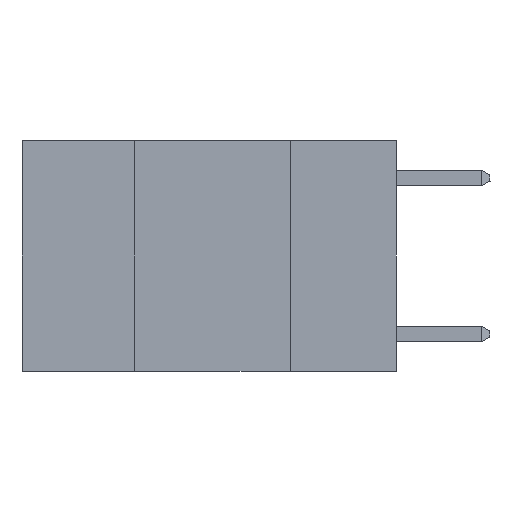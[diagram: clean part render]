
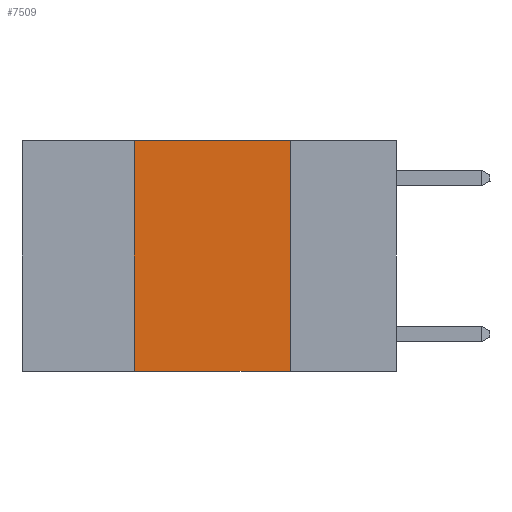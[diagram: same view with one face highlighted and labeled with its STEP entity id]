
A CAD part, left-side view. The second image highlights one B-rep face of the part: STEP entity #7509.
In plain terms, the highlighted planar face has unit normal (-1, 0, 0).
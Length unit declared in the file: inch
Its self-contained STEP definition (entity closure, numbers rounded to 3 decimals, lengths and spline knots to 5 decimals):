
#408 = ORIENTED_EDGE ( 'NONE', *, *, #969, .F. ) ;
#866 = LINE ( 'NONE', #1136, #2808 ) ;
#969 = EDGE_CURVE ( 'NONE', #2059, #5249, #866, .T. ) ;
#1136 = CARTESIAN_POINT ( 'NONE',  ( 0., 0.6, 0. ) ) ;
#1312 = AXIS2_PLACEMENT_3D ( 'NONE', #4613, #2188, #7841 ) ;
#1354 = PLANE ( 'NONE',  #1312 ) ;
#1768 = LINE ( 'NONE', #5942, #2265 ) ;
#2059 = VERTEX_POINT ( 'NONE', #3646 ) ;
#2148 = CARTESIAN_POINT ( 'NONE',  ( 0., 0.6, -0.37 ) ) ;
#2188 = DIRECTION ( 'NONE',  ( 1., 0., 0. ) ) ;
#2265 = VECTOR ( 'NONE', #7487, 39.37008 ) ;
#2636 = DIRECTION ( 'NONE',  ( 0., -1., 0. ) ) ;
#2808 = VECTOR ( 'NONE', #2636, 39.37008 ) ;
#3615 = CARTESIAN_POINT ( 'NONE',  ( 0., 0.42, -0.37 ) ) ;
#3646 = CARTESIAN_POINT ( 'NONE',  ( 0., 0.42, 0. ) ) ;
#4138 = CARTESIAN_POINT ( 'NONE',  ( 0., 0.17, 0. ) ) ;
#4613 = CARTESIAN_POINT ( 'NONE',  ( 0., 0.6, 0. ) ) ;
#5249 = VERTEX_POINT ( 'NONE', #4138 ) ;
#5309 = CARTESIAN_POINT ( 'NONE',  ( 0., 0.17, -0.37 ) ) ;
#5350 = EDGE_LOOP ( 'NONE', ( #9798, #408, #6287, #7419 ) ) ;
#5364 = EDGE_CURVE ( 'NONE', #5249, #6177, #1768, .T. ) ;
#5484 = VECTOR ( 'NONE', #7800, 39.37008 ) ;
#5546 = LINE ( 'NONE', #2148, #9553 ) ;
#5942 = CARTESIAN_POINT ( 'NONE',  ( 0., 0.17, 0. ) ) ;
#6177 = VERTEX_POINT ( 'NONE', #5309 ) ;
#6278 = EDGE_CURVE ( 'NONE', #9271, #2059, #7575, .T. ) ;
#6287 = ORIENTED_EDGE ( 'NONE', *, *, #6278, .F. ) ;
#6983 = CARTESIAN_POINT ( 'NONE',  ( 0., 0.42, 0. ) ) ;
#7419 = ORIENTED_EDGE ( 'NONE', *, *, #8772, .T. ) ;
#7487 = DIRECTION ( 'NONE',  ( 0., 0., -1. ) ) ;
#7509 = ADVANCED_FACE ( 'NONE', ( #8329 ), #1354, .F. ) ;
#7575 = LINE ( 'NONE', #6983, #5484 ) ;
#7800 = DIRECTION ( 'NONE',  ( 0., 0., 1. ) ) ;
#7841 = DIRECTION ( 'NONE',  ( 0., 0., -1. ) ) ;
#8329 = FACE_OUTER_BOUND ( 'NONE', #5350, .T. ) ;
#8772 = EDGE_CURVE ( 'NONE', #9271, #6177, #5546, .T. ) ;
#9271 = VERTEX_POINT ( 'NONE', #3615 ) ;
#9429 = DIRECTION ( 'NONE',  ( 0., -1., 0. ) ) ;
#9553 = VECTOR ( 'NONE', #9429, 39.37008 ) ;
#9798 = ORIENTED_EDGE ( 'NONE', *, *, #5364, .F. ) ;
